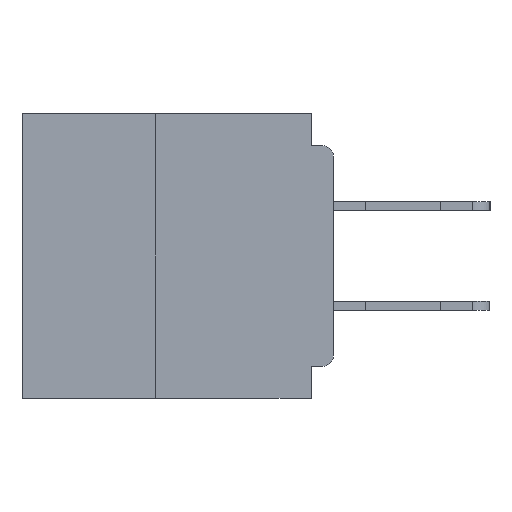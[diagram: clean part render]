
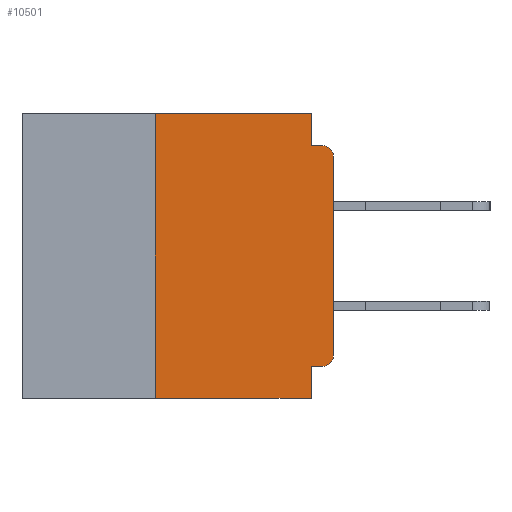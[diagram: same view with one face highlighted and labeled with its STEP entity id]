
A CAD part, left-side view. The second image highlights one B-rep face of the part: STEP entity #10501.
In plain terms, the highlighted planar face has unit normal (-1, 0, 0).
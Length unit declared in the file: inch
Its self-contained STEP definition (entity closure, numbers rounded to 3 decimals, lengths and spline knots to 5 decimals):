
#312 = VERTEX_POINT ( 'NONE', #28768 ) ;
#432 = CARTESIAN_POINT ( 'NONE',  ( 0., 0.437, -0.4 ) ) ;
#1332 = ORIENTED_EDGE ( 'NONE', *, *, #4194, .F. ) ;
#1345 = EDGE_LOOP ( 'NONE', ( #36200, #21318, #30124, #15199, #8955, #18231, #13444, #19222, #1332, #3584 ) ) ;
#1785 = EDGE_CURVE ( 'NONE', #39542, #17383, #16334, .T. ) ;
#1895 = EDGE_CURVE ( 'NONE', #4986, #39542, #29866, .T. ) ;
#3088 = VECTOR ( 'NONE', #24896, 39.37008 ) ;
#3584 = ORIENTED_EDGE ( 'NONE', *, *, #8981, .T. ) ;
#3811 = LINE ( 'NONE', #432, #27547 ) ;
#3897 = PLANE ( 'NONE',  #19107 ) ;
#3969 = DIRECTION ( 'NONE',  ( -1., 0., 0. ) ) ;
#4194 = EDGE_CURVE ( 'NONE', #19988, #39993, #29257, .T. ) ;
#4664 = VECTOR ( 'NONE', #15636, 39.37008 ) ;
#4986 = VERTEX_POINT ( 'NONE', #6119 ) ;
#5066 = DIRECTION ( 'NONE',  ( 0., 0., 1. ) ) ;
#6119 = CARTESIAN_POINT ( 'NONE',  ( 0., 0.25, -0.4 ) ) ;
#6752 = DIRECTION ( 'NONE',  ( 0., -1., 0. ) ) ;
#7598 = DIRECTION ( 'NONE',  ( -1., 0., 0. ) ) ;
#8109 = VECTOR ( 'NONE', #23743, 39.37008 ) ;
#8765 = DIRECTION ( 'NONE',  ( 0., 0., -1. ) ) ;
#8955 = ORIENTED_EDGE ( 'NONE', *, *, #1785, .F. ) ;
#8981 = EDGE_CURVE ( 'NONE', #19988, #11294, #21838, .T. ) ;
#9620 = CARTESIAN_POINT ( 'NONE',  ( 0., 0.25, -0.4 ) ) ;
#10132 = CARTESIAN_POINT ( 'NONE',  ( 0., 0., -0.355 ) ) ;
#10162 = DIRECTION ( 'NONE',  ( 0., 1., 0. ) ) ;
#10190 = DIRECTION ( 'NONE',  ( 0., 0., -1. ) ) ;
#10501 = ADVANCED_FACE ( 'NONE', ( #32360 ), #3897, .F. ) ;
#11294 = VERTEX_POINT ( 'NONE', #23093 ) ;
#11751 = EDGE_CURVE ( 'NONE', #11294, #312, #25932, .T. ) ;
#11941 = CARTESIAN_POINT ( 'NONE',  ( 0., 0.031, 0. ) ) ;
#12102 = AXIS2_PLACEMENT_3D ( 'NONE', #26061, #7598, #29221 ) ;
#12470 = VECTOR ( 'NONE', #5066, 39.37008 ) ;
#12824 = DIRECTION ( 'NONE',  ( 0., 0., 1. ) ) ;
#13364 = CARTESIAN_POINT ( 'NONE',  ( 0., 0.015, -0.045 ) ) ;
#13444 = ORIENTED_EDGE ( 'NONE', *, *, #31821, .T. ) ;
#15199 = ORIENTED_EDGE ( 'NONE', *, *, #20690, .F. ) ;
#15345 = VERTEX_POINT ( 'NONE', #23970 ) ;
#15408 = VECTOR ( 'NONE', #8765, 39.37008 ) ;
#15636 = DIRECTION ( 'NONE',  ( 0., 0., -1. ) ) ;
#16334 = LINE ( 'NONE', #24737, #8109 ) ;
#16374 = LINE ( 'NONE', #11941, #15408 ) ;
#17383 = VERTEX_POINT ( 'NONE', #36404 ) ;
#18231 = ORIENTED_EDGE ( 'NONE', *, *, #1895, .F. ) ;
#19107 = AXIS2_PLACEMENT_3D ( 'NONE', #25556, #28688, #10190 ) ;
#19147 = EDGE_CURVE ( 'NONE', #312, #25587, #24203, .T. ) ;
#19222 = ORIENTED_EDGE ( 'NONE', *, *, #21454, .F. ) ;
#19988 = VERTEX_POINT ( 'NONE', #39264 ) ;
#20690 = EDGE_CURVE ( 'NONE', #17383, #15345, #16374, .T. ) ;
#21318 = ORIENTED_EDGE ( 'NONE', *, *, #19147, .T. ) ;
#21454 = EDGE_CURVE ( 'NONE', #39993, #38351, #29361, .T. ) ;
#21803 = CARTESIAN_POINT ( 'NONE',  ( 0., 0., -0.045 ) ) ;
#21838 = CIRCLE ( 'NONE', #12102, 0.015 ) ;
#22515 = CARTESIAN_POINT ( 'NONE',  ( 0., 0.015, -0.06 ) ) ;
#22765 = EDGE_CURVE ( 'NONE', #15345, #25587, #27815, .T. ) ;
#23093 = CARTESIAN_POINT ( 'NONE',  ( 0., 0., -0.34 ) ) ;
#23743 = DIRECTION ( 'NONE',  ( 0., -1., 0. ) ) ;
#23970 = CARTESIAN_POINT ( 'NONE',  ( 0., 0.031, -0.045 ) ) ;
#24203 = CIRCLE ( 'NONE', #29959, 0.015 ) ;
#24737 = CARTESIAN_POINT ( 'NONE',  ( 0., 0.437, 0. ) ) ;
#24896 = DIRECTION ( 'NONE',  ( 0., -1., 0. ) ) ;
#25556 = CARTESIAN_POINT ( 'NONE',  ( 0., 0.437, 0. ) ) ;
#25587 = VERTEX_POINT ( 'NONE', #13364 ) ;
#25613 = DIRECTION ( 'NONE',  ( 0., 0., -1. ) ) ;
#25932 = LINE ( 'NONE', #37425, #34162 ) ;
#26061 = CARTESIAN_POINT ( 'NONE',  ( 0., 0.015, -0.34 ) ) ;
#27547 = VECTOR ( 'NONE', #6752, 39.37008 ) ;
#27815 = LINE ( 'NONE', #21803, #3088 ) ;
#27859 = CARTESIAN_POINT ( 'NONE',  ( 0., 0.031, -0.355 ) ) ;
#28261 = VECTOR ( 'NONE', #10162, 39.37008 ) ;
#28310 = CARTESIAN_POINT ( 'NONE',  ( 0., 0.25, 0. ) ) ;
#28688 = DIRECTION ( 'NONE',  ( 1., 0., 0. ) ) ;
#28768 = CARTESIAN_POINT ( 'NONE',  ( 0., 0., -0.06 ) ) ;
#29221 = DIRECTION ( 'NONE',  ( 0., 0., -1. ) ) ;
#29257 = LINE ( 'NONE', #10132, #28261 ) ;
#29361 = LINE ( 'NONE', #37146, #4664 ) ;
#29866 = LINE ( 'NONE', #9620, #12470 ) ;
#29959 = AXIS2_PLACEMENT_3D ( 'NONE', #22515, #3969, #25613 ) ;
#30124 = ORIENTED_EDGE ( 'NONE', *, *, #22765, .F. ) ;
#31821 = EDGE_CURVE ( 'NONE', #4986, #38351, #3811, .T. ) ;
#32360 = FACE_OUTER_BOUND ( 'NONE', #1345, .T. ) ;
#34162 = VECTOR ( 'NONE', #12824, 39.37008 ) ;
#34667 = CARTESIAN_POINT ( 'NONE',  ( 0., 0.031, -0.4 ) ) ;
#36200 = ORIENTED_EDGE ( 'NONE', *, *, #11751, .T. ) ;
#36404 = CARTESIAN_POINT ( 'NONE',  ( 0., 0.031, 0. ) ) ;
#37146 = CARTESIAN_POINT ( 'NONE',  ( 0., 0.031, -0.4 ) ) ;
#37425 = CARTESIAN_POINT ( 'NONE',  ( 0., 0., 0. ) ) ;
#38351 = VERTEX_POINT ( 'NONE', #34667 ) ;
#39264 = CARTESIAN_POINT ( 'NONE',  ( 0., 0.015, -0.355 ) ) ;
#39542 = VERTEX_POINT ( 'NONE', #28310 ) ;
#39993 = VERTEX_POINT ( 'NONE', #27859 ) ;
